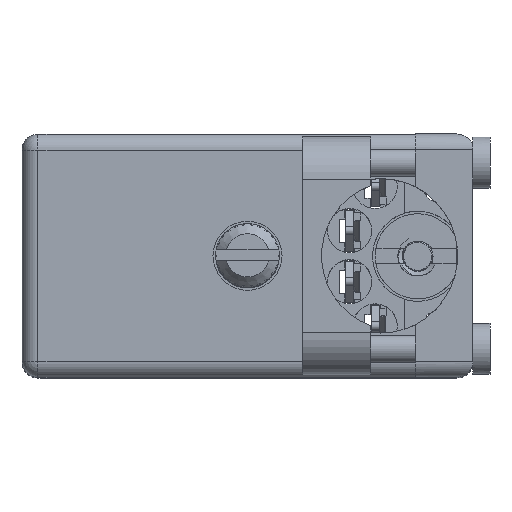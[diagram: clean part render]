
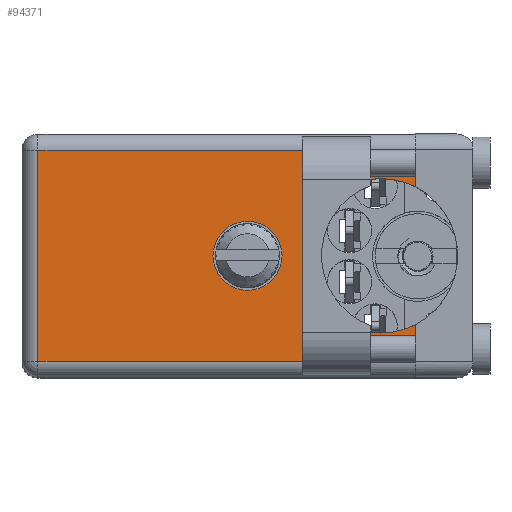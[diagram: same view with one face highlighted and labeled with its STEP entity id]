
A CAD part, top view. The second image highlights one B-rep face of the part: STEP entity #94371.
In plain terms, the highlighted face is planar.
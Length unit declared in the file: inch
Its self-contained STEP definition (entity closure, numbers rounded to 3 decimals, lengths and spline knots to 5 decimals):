
#135 = EDGE_CURVE ( 'NONE', #122195, #84246, #165840, .T. ) ;
#5653 = EDGE_CURVE ( 'NONE', #152459, #19403, #124514, .T. ) ;
#9335 = ORIENTED_EDGE ( 'NONE', *, *, #137701, .F. ) ;
#16302 = CARTESIAN_POINT ( 'NONE',  ( 1.155, 0.906, -0.047 ) ) ;
#18943 = DIRECTION ( 'NONE',  ( 0., 0., 1. ) ) ;
#19403 = VERTEX_POINT ( 'NONE', #159307 ) ;
#20514 = CARTESIAN_POINT ( 'NONE',  ( 0.6625, 0.906, -0.256 ) ) ;
#23144 = CARTESIAN_POINT ( 'NONE',  ( 0.047, 0.906, -0.715 ) ) ;
#26811 = CIRCLE ( 'NONE', #155863, 0.1015 ) ;
#27933 = CARTESIAN_POINT ( 'NONE',  ( 1.155, 0.906, -0.15471 ) ) ;
#29194 = CARTESIAN_POINT ( 'NONE',  ( 1.155, 0.906, -0.56029 ) ) ;
#34004 = CARTESIAN_POINT ( 'NONE',  ( 0.047, 0.906, -0.668 ) ) ;
#34161 = CIRCLE ( 'NONE', #104839, 0.227 ) ;
#34277 = CARTESIAN_POINT ( 'NONE',  ( 1.155, 0.906, -0.668 ) ) ;
#34689 = CARTESIAN_POINT ( 'NONE',  ( 0.047, 0.906, -0.047 ) ) ;
#35571 = EDGE_CURVE ( 'NONE', #84246, #152459, #34161, .T. ) ;
#36739 = CARTESIAN_POINT ( 'NONE',  ( 1.053, 0.906, -0.3575 ) ) ;
#39235 = VERTEX_POINT ( 'NONE', #86122 ) ;
#39325 = CARTESIAN_POINT ( 'NONE',  ( 0., 0.906, -0.668 ) ) ;
#40521 = VECTOR ( 'NONE', #146580, 39.37008 ) ;
#42157 = ORIENTED_EDGE ( 'NONE', *, *, #89087, .F. ) ;
#50047 = VERTEX_POINT ( 'NONE', #34004 ) ;
#50066 = DIRECTION ( 'NONE',  ( 0., 1., 0. ) ) ;
#55444 = EDGE_LOOP ( 'NONE', ( #116231, #69421, #56869, #65747, #57702, #78646, #95198, #57788 ) ) ;
#56869 = ORIENTED_EDGE ( 'NONE', *, *, #156987, .T. ) ;
#57702 = ORIENTED_EDGE ( 'NONE', *, *, #5653, .F. ) ;
#57788 = ORIENTED_EDGE ( 'NONE', *, *, #99087, .F. ) ;
#60365 = LINE ( 'NONE', #16302, #137074 ) ;
#62347 = VERTEX_POINT ( 'NONE', #29194 ) ;
#65747 = ORIENTED_EDGE ( 'NONE', *, *, #115309, .T. ) ;
#66222 = DIRECTION ( 'NONE',  ( 0., 1., 0. ) ) ;
#69421 = ORIENTED_EDGE ( 'NONE', *, *, #80609, .T. ) ;
#74054 = VECTOR ( 'NONE', #120302, 39.37008 ) ;
#75227 = DIRECTION ( 'NONE',  ( 0., 0., 1. ) ) ;
#78603 = EDGE_LOOP ( 'NONE', ( #9335, #42157 ) ) ;
#78646 = ORIENTED_EDGE ( 'NONE', *, *, #35571, .F. ) ;
#80609 = EDGE_CURVE ( 'NONE', #160891, #50047, #150989, .T. ) ;
#82263 = CIRCLE ( 'NONE', #169261, 0.1015 ) ;
#84246 = VERTEX_POINT ( 'NONE', #120508 ) ;
#85839 = CARTESIAN_POINT ( 'NONE',  ( 1.053, 0.906, -0.5845 ) ) ;
#86122 = CARTESIAN_POINT ( 'NONE',  ( 0.6625, 0.906, -0.459 ) ) ;
#89087 = EDGE_CURVE ( 'NONE', #39235, #166757, #82263, .T. ) ;
#90349 = CARTESIAN_POINT ( 'NONE',  ( 0., 0.906, -0.715 ) ) ;
#94371 = ADVANCED_FACE ( 'NONE', ( #171960, #97566 ), #119211, .T. ) ;
#95198 = ORIENTED_EDGE ( 'NONE', *, *, #135, .F. ) ;
#97286 = AXIS2_PLACEMENT_3D ( 'NONE', #36739, #66222, #173481 ) ;
#97566 = FACE_BOUND ( 'NONE', #78603, .T. ) ;
#98660 = VECTOR ( 'NONE', #177354, 39.37008 ) ;
#99087 = EDGE_CURVE ( 'NONE', #62347, #122195, #185691, .T. ) ;
#104839 = AXIS2_PLACEMENT_3D ( 'NONE', #124848, #185190, #153054 ) ;
#106274 = CARTESIAN_POINT ( 'NONE',  ( 1.053, 0.906, -0.3575 ) ) ;
#107602 = DIRECTION ( 'NONE',  ( 0., 1., 0. ) ) ;
#115309 = EDGE_CURVE ( 'NONE', #153909, #19403, #60365, .T. ) ;
#116231 = ORIENTED_EDGE ( 'NONE', *, *, #141667, .F. ) ;
#116998 = AXIS2_PLACEMENT_3D ( 'NONE', #90349, #180865, #152029 ) ;
#119211 = PLANE ( 'NONE',  #116998 ) ;
#120302 = DIRECTION ( 'NONE',  ( 0., 0., 1. ) ) ;
#120508 = CARTESIAN_POINT ( 'NONE',  ( 1.053, 0.906, -0.1305 ) ) ;
#122195 = VERTEX_POINT ( 'NONE', #85839 ) ;
#124514 = LINE ( 'NONE', #196001, #74054 ) ;
#124848 = CARTESIAN_POINT ( 'NONE',  ( 1.053, 0.906, -0.3575 ) ) ;
#125600 = DIRECTION ( 'NONE',  ( 1., 0., 0. ) ) ;
#137074 = VECTOR ( 'NONE', #125600, 39.37008 ) ;
#137701 = EDGE_CURVE ( 'NONE', #166757, #39235, #26811, .T. ) ;
#141667 = EDGE_CURVE ( 'NONE', #160891, #62347, #168006, .T. ) ;
#141837 = CARTESIAN_POINT ( 'NONE',  ( 0.6625, 0.906, -0.3575 ) ) ;
#144163 = LINE ( 'NONE', #23144, #98660 ) ;
#146580 = DIRECTION ( 'NONE',  ( -1., 0., 0. ) ) ;
#150989 = LINE ( 'NONE', #39325, #40521 ) ;
#152029 = DIRECTION ( 'NONE',  ( 0., 0., 1. ) ) ;
#152459 = VERTEX_POINT ( 'NONE', #27933 ) ;
#153054 = DIRECTION ( 'NONE',  ( 0., 0., 1. ) ) ;
#153909 = VERTEX_POINT ( 'NONE', #34689 ) ;
#155863 = AXIS2_PLACEMENT_3D ( 'NONE', #167141, #198579, #75227 ) ;
#156987 = EDGE_CURVE ( 'NONE', #50047, #153909, #144163, .T. ) ;
#159307 = CARTESIAN_POINT ( 'NONE',  ( 1.155, 0.906, -0.047 ) ) ;
#160725 = VECTOR ( 'NONE', #190815, 39.37008 ) ;
#160891 = VERTEX_POINT ( 'NONE', #34277 ) ;
#165840 = CIRCLE ( 'NONE', #179969, 0.227 ) ;
#166757 = VERTEX_POINT ( 'NONE', #20514 ) ;
#167141 = CARTESIAN_POINT ( 'NONE',  ( 0.6625, 0.906, -0.3575 ) ) ;
#168006 = LINE ( 'NONE', #174737, #160725 ) ;
#169261 = AXIS2_PLACEMENT_3D ( 'NONE', #141837, #50066, #172710 ) ;
#171960 = FACE_OUTER_BOUND ( 'NONE', #55444, .T. ) ;
#172710 = DIRECTION ( 'NONE',  ( 0., 0., 1. ) ) ;
#173481 = DIRECTION ( 'NONE',  ( 0., 0., 1. ) ) ;
#174737 = CARTESIAN_POINT ( 'NONE',  ( 1.155, 0.906, 0. ) ) ;
#177354 = DIRECTION ( 'NONE',  ( 0., 0., 1. ) ) ;
#179969 = AXIS2_PLACEMENT_3D ( 'NONE', #106274, #107602, #18943 ) ;
#180865 = DIRECTION ( 'NONE',  ( 0., 1., 0. ) ) ;
#185190 = DIRECTION ( 'NONE',  ( 0., 1., 0. ) ) ;
#185691 = CIRCLE ( 'NONE', #97286, 0.227 ) ;
#190815 = DIRECTION ( 'NONE',  ( 0., 0., 1. ) ) ;
#196001 = CARTESIAN_POINT ( 'NONE',  ( 1.155, 0.906, 0. ) ) ;
#198579 = DIRECTION ( 'NONE',  ( 0., 1., 0. ) ) ;
